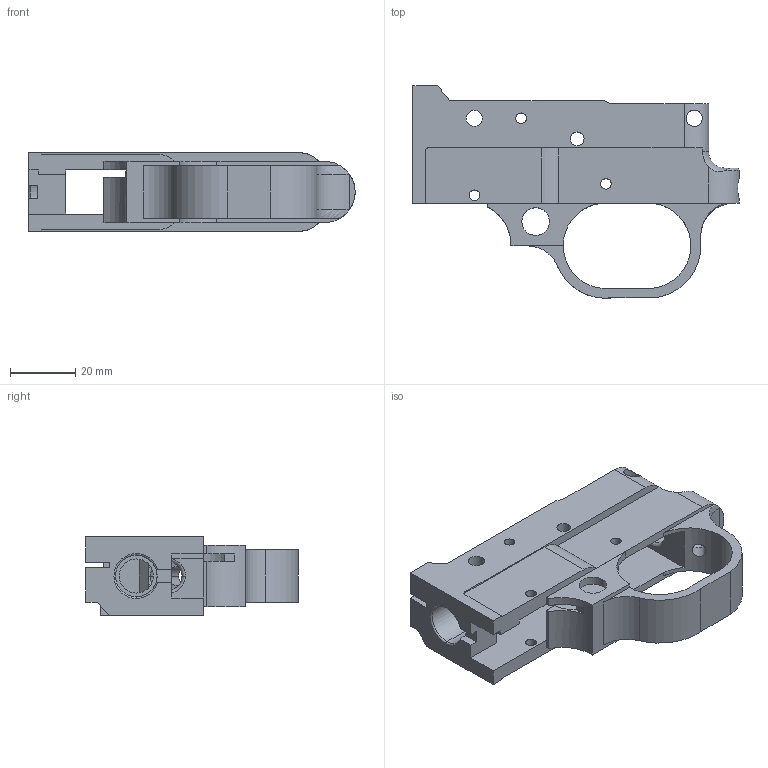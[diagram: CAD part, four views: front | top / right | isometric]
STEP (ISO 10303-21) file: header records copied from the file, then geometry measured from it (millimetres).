
FILE_DESCRIPTION (( 'STEP AP214' ), '1' );
FILE_NAME ('10-22 trigger 4-2.STEP', '2015-05-08T20:11:45', ( 'WarFairy' ), ( '' ), 'SwSTEP 2.0', 'SolidWorks 2015', '' );
FILE_SCHEMA (( 'AUTOMOTIVE_DESIGN' ));
Length unit declared in the file: millimetre
Products named in the file (1): 10-22 trigger 4-2
Bounding box: 100.08 x 65.17 x 24 mm (x, y, z)
Volume: 37487.5 mm3; surface area: 21489.2 mm2
Topology: 1 solids, 1 shells, 133 faces, 391 edges, 254 vertices
Faces by surface type: plane 66, cylinder 55, torus 8, bspline 4
Entity records: 5043 total; most frequent: CARTESIAN_POINT 1353, ORIENTED_EDGE 782, DIRECTION 757, EDGE_CURVE 391, AXIS2_PLACEMENT_3D 264, VERTEX_POINT 254, LINE 229, VECTOR 229
